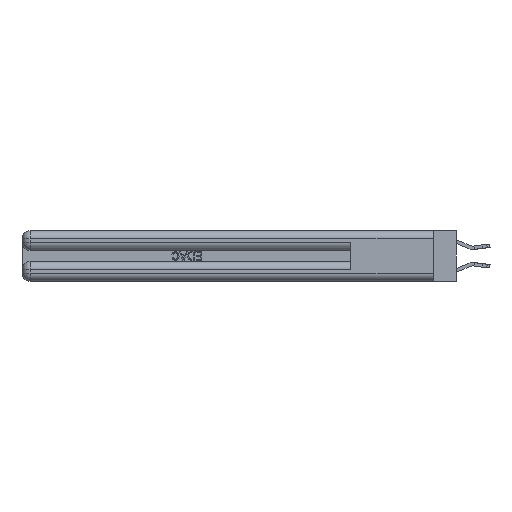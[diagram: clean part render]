
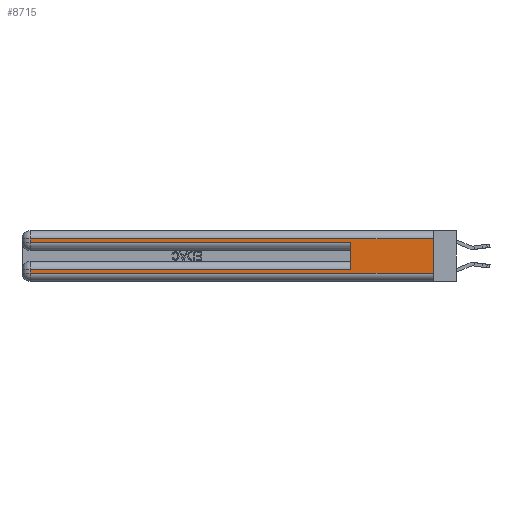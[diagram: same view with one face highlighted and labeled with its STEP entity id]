
A CAD part, left-side view. The second image highlights one B-rep face of the part: STEP entity #8715.
In plain terms, the highlighted planar face has unit normal (-1, 0, 0).
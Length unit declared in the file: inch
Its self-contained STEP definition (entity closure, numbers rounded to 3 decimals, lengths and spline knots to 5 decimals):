
#478 = CARTESIAN_POINT ( 'NONE',  ( 0., 0.6, 0.145 ) ) ;
#2321 = EDGE_CURVE ( 'NONE', #21115, #30463, #18973, .T. ) ;
#2342 = VERTEX_POINT ( 'NONE', #21643 ) ;
#2435 = EDGE_CURVE ( 'NONE', #11739, #14916, #22397, .T. ) ;
#2856 = ORIENTED_EDGE ( 'NONE', *, *, #2321, .F. ) ;
#3225 = LINE ( 'NONE', #24645, #13983 ) ;
#3892 = ORIENTED_EDGE ( 'NONE', *, *, #27037, .T. ) ;
#3909 = CARTESIAN_POINT ( 'NONE',  ( 0., 2.94, 0.06 ) ) ;
#4032 = FACE_OUTER_BOUND ( 'NONE', #12910, .T. ) ;
#4212 = VECTOR ( 'NONE', #24420, 39.37008 ) ;
#4529 = DIRECTION ( 'NONE',  ( 0., 1., 0. ) ) ;
#4775 = VERTEX_POINT ( 'NONE', #17378 ) ;
#4962 = LINE ( 'NONE', #15737, #26790 ) ;
#6600 = ORIENTED_EDGE ( 'NONE', *, *, #24702, .T. ) ;
#6671 = CARTESIAN_POINT ( 'NONE',  ( 0., 0., 0.285 ) ) ;
#6841 = VECTOR ( 'NONE', #16192, 39.37008 ) ;
#6958 = VERTEX_POINT ( 'NONE', #26780 ) ;
#7260 = CARTESIAN_POINT ( 'NONE',  ( 0., 0., 0.37 ) ) ;
#7657 = VERTEX_POINT ( 'NONE', #3909 ) ;
#8640 = CARTESIAN_POINT ( 'NONE',  ( 0., 2.94, 0.285 ) ) ;
#8715 = ADVANCED_FACE ( 'NONE', ( #4032 ), #26079, .F. ) ;
#9063 = DIRECTION ( 'NONE',  ( 1., 0., 0. ) ) ;
#9495 = CARTESIAN_POINT ( 'NONE',  ( 0., 0., 0.31 ) ) ;
#10194 = ORIENTED_EDGE ( 'NONE', *, *, #21030, .T. ) ;
#11739 = VERTEX_POINT ( 'NONE', #19529 ) ;
#12057 = LINE ( 'NONE', #26723, #23728 ) ;
#12614 = CARTESIAN_POINT ( 'NONE',  ( 0., 0., 0.06 ) ) ;
#12910 = EDGE_LOOP ( 'NONE', ( #2856, #25757, #19611, #10194, #25257, #6600, #3892, #23684 ) ) ;
#13983 = VECTOR ( 'NONE', #17447, 39.37008 ) ;
#14582 = CARTESIAN_POINT ( 'NONE',  ( 0., 2.94, 0.37 ) ) ;
#14916 = VERTEX_POINT ( 'NONE', #8640 ) ;
#14979 = VECTOR ( 'NONE', #28980, 39.37008 ) ;
#15737 = CARTESIAN_POINT ( 'NONE',  ( 0., 0., 0.31 ) ) ;
#15898 = VECTOR ( 'NONE', #4529, 39.37008 ) ;
#16192 = DIRECTION ( 'NONE',  ( 0., -1., 0. ) ) ;
#17038 = DIRECTION ( 'NONE',  ( 0., -1., 0. ) ) ;
#17378 = CARTESIAN_POINT ( 'NONE',  ( 0., 2.94, 0.085 ) ) ;
#17447 = DIRECTION ( 'NONE',  ( 0., 0., -1. ) ) ;
#18398 = DIRECTION ( 'NONE',  ( 0., 0., -1. ) ) ;
#18559 = AXIS2_PLACEMENT_3D ( 'NONE', #28115, #9063, #18398 ) ;
#18742 = EDGE_CURVE ( 'NONE', #7657, #30463, #12057, .T. ) ;
#18817 = DIRECTION ( 'NONE',  ( 0., 0., -1. ) ) ;
#18973 = LINE ( 'NONE', #7260, #27094 ) ;
#19529 = CARTESIAN_POINT ( 'NONE',  ( 0., 2.94, 0.31 ) ) ;
#19611 = ORIENTED_EDGE ( 'NONE', *, *, #2435, .T. ) ;
#20595 = EDGE_CURVE ( 'NONE', #21115, #11739, #4962, .T. ) ;
#21030 = EDGE_CURVE ( 'NONE', #14916, #2342, #28086, .T. ) ;
#21115 = VERTEX_POINT ( 'NONE', #9495 ) ;
#21643 = CARTESIAN_POINT ( 'NONE',  ( 0., 0.6, 0.285 ) ) ;
#22397 = LINE ( 'NONE', #14582, #4212 ) ;
#23684 = ORIENTED_EDGE ( 'NONE', *, *, #18742, .T. ) ;
#23728 = VECTOR ( 'NONE', #17038, 39.37008 ) ;
#24420 = DIRECTION ( 'NONE',  ( 0., 0., -1. ) ) ;
#24645 = CARTESIAN_POINT ( 'NONE',  ( 0., 2.94, 0.37 ) ) ;
#24702 = EDGE_CURVE ( 'NONE', #6958, #4775, #25790, .T. ) ;
#25257 = ORIENTED_EDGE ( 'NONE', *, *, #27285, .F. ) ;
#25757 = ORIENTED_EDGE ( 'NONE', *, *, #20595, .T. ) ;
#25790 = LINE ( 'NONE', #28288, #15898 ) ;
#26079 = PLANE ( 'NONE',  #18559 ) ;
#26315 = LINE ( 'NONE', #478, #14979 ) ;
#26723 = CARTESIAN_POINT ( 'NONE',  ( 0., 0., 0.06 ) ) ;
#26780 = CARTESIAN_POINT ( 'NONE',  ( 0., 0.6, 0.085 ) ) ;
#26790 = VECTOR ( 'NONE', #27306, 39.37008 ) ;
#27037 = EDGE_CURVE ( 'NONE', #4775, #7657, #3225, .T. ) ;
#27094 = VECTOR ( 'NONE', #18817, 39.37008 ) ;
#27285 = EDGE_CURVE ( 'NONE', #6958, #2342, #26315, .T. ) ;
#27306 = DIRECTION ( 'NONE',  ( 0., 1., 0. ) ) ;
#28086 = LINE ( 'NONE', #6671, #6841 ) ;
#28115 = CARTESIAN_POINT ( 'NONE',  ( 0., 0., 0.37 ) ) ;
#28288 = CARTESIAN_POINT ( 'NONE',  ( 0., 0., 0.085 ) ) ;
#28980 = DIRECTION ( 'NONE',  ( 0., 0., 1. ) ) ;
#30463 = VERTEX_POINT ( 'NONE', #12614 ) ;
